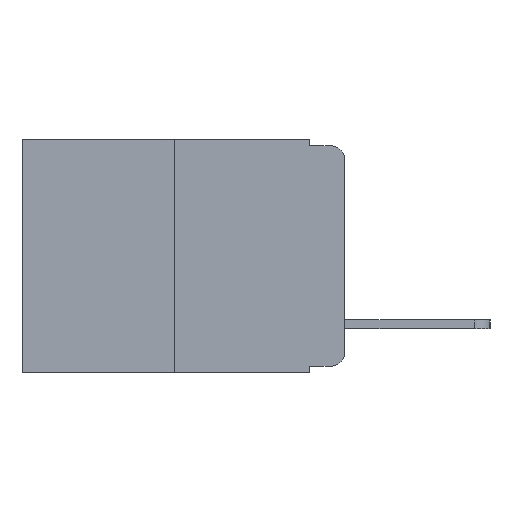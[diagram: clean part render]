
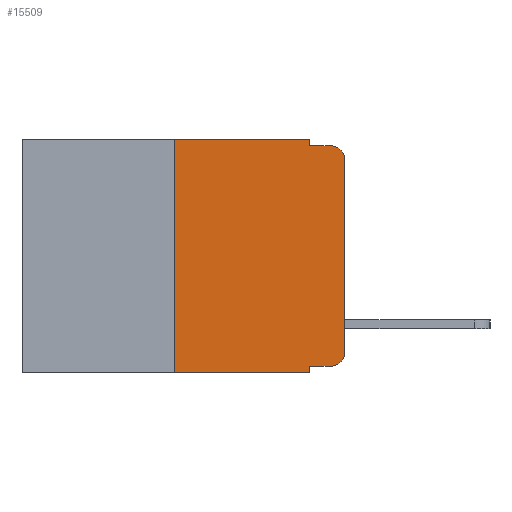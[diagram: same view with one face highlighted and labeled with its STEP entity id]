
A CAD part, left-side view. The second image highlights one B-rep face of the part: STEP entity #15509.
In plain terms, the highlighted planar face has unit normal (-1, 0, 0).
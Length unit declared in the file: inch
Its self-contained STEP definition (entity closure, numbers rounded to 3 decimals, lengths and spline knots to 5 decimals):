
#57 = CARTESIAN_POINT ( 'NONE',  ( 0., 0.25, -0.343 ) ) ;
#209 = LINE ( 'NONE', #6267, #4239 ) ;
#348 = VERTEX_POINT ( 'NONE', #15054 ) ;
#390 = CARTESIAN_POINT ( 'NONE',  ( 0., 0.25, 0. ) ) ;
#716 = VERTEX_POINT ( 'NONE', #2561 ) ;
#778 = EDGE_CURVE ( 'NONE', #8616, #9093, #8417, .T. ) ;
#810 = CARTESIAN_POINT ( 'NONE',  ( 0., 0.051, -0.333 ) ) ;
#820 = DIRECTION ( 'NONE',  ( 0., -1., 0. ) ) ;
#971 = VECTOR ( 'NONE', #15586, 39.37008 ) ;
#1055 = DIRECTION ( 'NONE',  ( 0., 0., 1. ) ) ;
#1162 = ORIENTED_EDGE ( 'NONE', *, *, #15246, .T. ) ;
#1406 = LINE ( 'NONE', #14428, #971 ) ;
#1430 = CARTESIAN_POINT ( 'NONE',  ( 0., 0.02, -0.313 ) ) ;
#1572 = ORIENTED_EDGE ( 'NONE', *, *, #8829, .T. ) ;
#2220 = AXIS2_PLACEMENT_3D ( 'NONE', #12108, #4589, #13338 ) ;
#2240 = ORIENTED_EDGE ( 'NONE', *, *, #778, .T. ) ;
#2561 = CARTESIAN_POINT ( 'NONE',  ( 0., 0., -0.313 ) ) ;
#2806 = DIRECTION ( 'NONE',  ( 0., 0., -1. ) ) ;
#2974 = VECTOR ( 'NONE', #1055, 39.37008 ) ;
#3298 = DIRECTION ( 'NONE',  ( 0., 0., -1. ) ) ;
#3410 = LINE ( 'NONE', #11366, #2974 ) ;
#4054 = EDGE_CURVE ( 'NONE', #13488, #9093, #8765, .T. ) ;
#4239 = VECTOR ( 'NONE', #13730, 39.37008 ) ;
#4424 = CARTESIAN_POINT ( 'NONE',  ( 0., 0.051, -0.333 ) ) ;
#4468 = DIRECTION ( 'NONE',  ( 0., -1., 0. ) ) ;
#4531 = DIRECTION ( 'NONE',  ( 0., 0., -1. ) ) ;
#4589 = DIRECTION ( 'NONE',  ( -1., 0., 0. ) ) ;
#4655 = PLANE ( 'NONE',  #7884 ) ;
#4937 = ORIENTED_EDGE ( 'NONE', *, *, #9969, .F. ) ;
#5032 = VERTEX_POINT ( 'NONE', #11796 ) ;
#5065 = VECTOR ( 'NONE', #820, 39.37008 ) ;
#5457 = EDGE_CURVE ( 'NONE', #5032, #6740, #1406, .T. ) ;
#5612 = VERTEX_POINT ( 'NONE', #6147 ) ;
#5705 = LINE ( 'NONE', #4424, #11961 ) ;
#5950 = DIRECTION ( 'NONE',  ( 1., 0., 0. ) ) ;
#6147 = CARTESIAN_POINT ( 'NONE',  ( 0., 0., -0.03 ) ) ;
#6267 = CARTESIAN_POINT ( 'NONE',  ( 0., 0.473, 0. ) ) ;
#6549 = DIRECTION ( 'NONE',  ( 0., 0., 1. ) ) ;
#6740 = VERTEX_POINT ( 'NONE', #15484 ) ;
#6790 = LINE ( 'NONE', #16447, #10119 ) ;
#7694 = CARTESIAN_POINT ( 'NONE',  ( 0., 0.051, -0.343 ) ) ;
#7884 = AXIS2_PLACEMENT_3D ( 'NONE', #13406, #5950, #14604 ) ;
#7907 = VECTOR ( 'NONE', #3298, 39.37008 ) ;
#8371 = CARTESIAN_POINT ( 'NONE',  ( 0., 0.051, 0. ) ) ;
#8417 = LINE ( 'NONE', #15480, #5065 ) ;
#8616 = VERTEX_POINT ( 'NONE', #57 ) ;
#8765 = LINE ( 'NONE', #10794, #12078 ) ;
#8829 = EDGE_CURVE ( 'NONE', #5612, #6740, #10772, .T. ) ;
#9093 = VERTEX_POINT ( 'NONE', #7694 ) ;
#9268 = ORIENTED_EDGE ( 'NONE', *, *, #5457, .F. ) ;
#9921 = EDGE_CURVE ( 'NONE', #10966, #348, #209, .T. ) ;
#9969 = EDGE_CURVE ( 'NONE', #8616, #10966, #3410, .T. ) ;
#10119 = VECTOR ( 'NONE', #6549, 39.37008 ) ;
#10421 = DIRECTION ( 'NONE',  ( -1., 0., 0. ) ) ;
#10423 = ORIENTED_EDGE ( 'NONE', *, *, #9921, .F. ) ;
#10772 = CIRCLE ( 'NONE', #2220, 0.02 ) ;
#10794 = CARTESIAN_POINT ( 'NONE',  ( 0., 0.051, 0. ) ) ;
#10966 = VERTEX_POINT ( 'NONE', #390 ) ;
#11005 = EDGE_LOOP ( 'NONE', ( #14264, #1572, #9268, #16211, #10423, #4937, #2240, #13148, #13905, #1162 ) ) ;
#11366 = CARTESIAN_POINT ( 'NONE',  ( 0., 0.25, 0. ) ) ;
#11551 = AXIS2_PLACEMENT_3D ( 'NONE', #1430, #10421, #2806 ) ;
#11622 = LINE ( 'NONE', #8371, #7907 ) ;
#11796 = CARTESIAN_POINT ( 'NONE',  ( 0., 0.051, -0.01 ) ) ;
#11961 = VECTOR ( 'NONE', #4468, 39.37008 ) ;
#11992 = CIRCLE ( 'NONE', #11551, 0.02 ) ;
#12078 = VECTOR ( 'NONE', #4531, 39.37008 ) ;
#12108 = CARTESIAN_POINT ( 'NONE',  ( 0., 0.02, -0.03 ) ) ;
#12171 = EDGE_CURVE ( 'NONE', #716, #5612, #6790, .T. ) ;
#12724 = VERTEX_POINT ( 'NONE', #16034 ) ;
#13148 = ORIENTED_EDGE ( 'NONE', *, *, #4054, .F. ) ;
#13338 = DIRECTION ( 'NONE',  ( 0., 0., -1. ) ) ;
#13406 = CARTESIAN_POINT ( 'NONE',  ( 0., 0.473, 0. ) ) ;
#13488 = VERTEX_POINT ( 'NONE', #810 ) ;
#13730 = DIRECTION ( 'NONE',  ( 0., -1., 0. ) ) ;
#13905 = ORIENTED_EDGE ( 'NONE', *, *, #16072, .T. ) ;
#14097 = EDGE_CURVE ( 'NONE', #348, #5032, #11622, .T. ) ;
#14259 = FACE_OUTER_BOUND ( 'NONE', #11005, .T. ) ;
#14264 = ORIENTED_EDGE ( 'NONE', *, *, #12171, .T. ) ;
#14428 = CARTESIAN_POINT ( 'NONE',  ( 0., 0.051, -0.01 ) ) ;
#14604 = DIRECTION ( 'NONE',  ( 0., 0., -1. ) ) ;
#15054 = CARTESIAN_POINT ( 'NONE',  ( 0., 0.051, 0. ) ) ;
#15246 = EDGE_CURVE ( 'NONE', #12724, #716, #11992, .T. ) ;
#15480 = CARTESIAN_POINT ( 'NONE',  ( 0., 0.473, -0.343 ) ) ;
#15484 = CARTESIAN_POINT ( 'NONE',  ( 0., 0.02, -0.01 ) ) ;
#15509 = ADVANCED_FACE ( 'NONE', ( #14259 ), #4655, .F. ) ;
#15586 = DIRECTION ( 'NONE',  ( 0., -1., 0. ) ) ;
#16034 = CARTESIAN_POINT ( 'NONE',  ( 0., 0.02, -0.333 ) ) ;
#16072 = EDGE_CURVE ( 'NONE', #13488, #12724, #5705, .T. ) ;
#16211 = ORIENTED_EDGE ( 'NONE', *, *, #14097, .F. ) ;
#16447 = CARTESIAN_POINT ( 'NONE',  ( 0., 0., 0. ) ) ;
